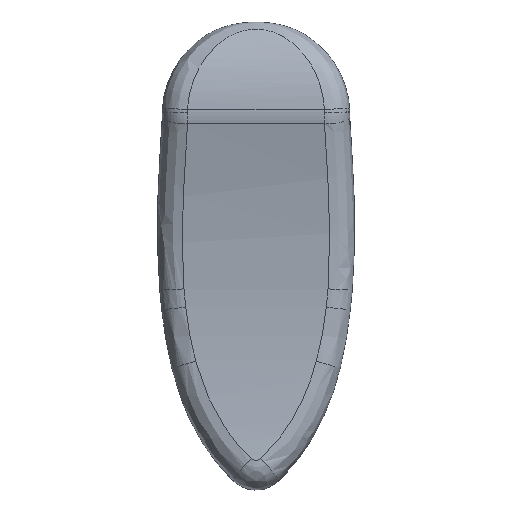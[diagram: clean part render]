
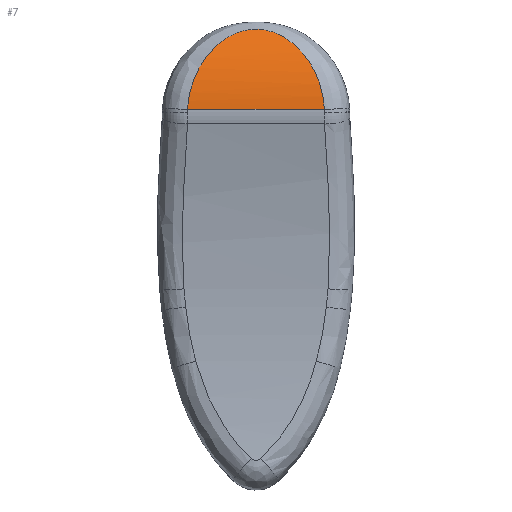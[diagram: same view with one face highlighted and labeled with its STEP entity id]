
A CAD part, top view. The second image highlights one B-rep face of the part: STEP entity #7.
In plain terms, the highlighted free-form (B-spline) face has degree [3, 1] with [4, 2] control points.
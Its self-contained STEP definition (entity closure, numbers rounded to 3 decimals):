
#7 = ADVANCED_FACE ( 'NONE', ( #804 ), #284, .T. ) ;
#9 = CARTESIAN_POINT ( 'NONE',  ( 25.436, 68.469, -62.998 ) ) ;
#22 = CARTESIAN_POINT ( 'NONE',  ( 2.512, 73.556, -64.651 ) ) ;
#30 = CARTESIAN_POINT ( 'NONE',  ( 16.093, 78.932, -67.916 ) ) ;
#35 = CARTESIAN_POINT ( 'NONE',  ( 23.451, 72.791, -64.319 ) ) ;
#46 = CARTESIAN_POINT ( 'NONE',  ( 8.005, 78.404, -67.486 ) ) ;
#100 = CARTESIAN_POINT ( 'NONE',  ( -0.837, 63.623, -62.366 ) ) ;
#114 = CARTESIAN_POINT ( 'NONE',  ( 0.157, 68.907, -63.109 ) ) ;
#131 = CARTESIAN_POINT ( 'NONE',  ( 22.933, 73.569, -64.646 ) ) ;
#135 = CARTESIAN_POINT ( 'NONE',  ( -1., 75.813, -65.048 ) ) ;
#139 = CARTESIAN_POINT ( 'NONE',  ( 21.771, 75.006, -65.341 ) ) ;
#147 = CARTESIAN_POINT ( 'NONE',  ( 26.431, 79.63, -68.522 ) ) ;
#168 = CARTESIAN_POINT ( 'NONE',  ( 5.312, 76.614, -66.253 ) ) ;
#174 = EDGE_CURVE ( 'NONE', #657, #1479, #650, .T. ) ;
#196 = ORIENTED_EDGE ( 'NONE', *, *, #174, .T. ) ;
#230 = ORIENTED_EDGE ( 'NONE', *, *, #1003, .T. ) ;
#237 = CARTESIAN_POINT ( 'NONE',  ( 20.806, 76.003, -65.887 ) ) ;
#256 = CARTESIAN_POINT ( 'NONE',  ( 11.724, 79.459, -68.368 ) ) ;
#281 = CARTESIAN_POINT ( 'NONE',  ( 10.259, 79.204, -68.145 ) ) ;
#284 = B_SPLINE_SURFACE_WITH_KNOTS ( 'NONE', 3, 1, ( 
 ( #831, #147 ),
 ( #135, #1433 ),
 ( #1033, #806 ),
 ( #1062, #907 ) ),
 .UNSPECIFIED., .F., .F., .F.,
 ( 4, 4 ),
 ( 2, 2 ),
 ( 0.236, 0.943 ),
 ( 0., 1. ),
 .UNSPECIFIED. ) ;
#294 = CARTESIAN_POINT ( 'NONE',  ( 10.745, 79.313, -68.24 ) ) ;
#302 = EDGE_LOOP ( 'NONE', ( #230, #196 ) ) ;
#311 = CARTESIAN_POINT ( 'NONE',  ( 4.277, 75.694, -65.701 ) ) ;
#388 = CARTESIAN_POINT ( 'NONE',  ( 25.703, 67.537, -62.809 ) ) ;
#393 = CARTESIAN_POINT ( 'NONE',  ( 8.856, 78.789, -67.796 ) ) ;
#426 = CARTESIAN_POINT ( 'NONE',  ( 19.033, 77.467, -66.804 ) ) ;
#501 = CARTESIAN_POINT ( 'NONE',  ( 0.005, 68.442, -63.004 ) ) ;
#526 = CARTESIAN_POINT ( 'NONE',  ( 26.097, 65.601, -62.517 ) ) ;
#529 = CARTESIAN_POINT ( 'NONE',  ( 26.268, 63.623, -62.366 ) ) ;
#536 = CARTESIAN_POINT ( 'NONE',  ( 5.674, 76.907, -66.439 ) ) ;
#627 = CARTESIAN_POINT ( 'NONE',  ( 22.072, 74.657, -65.164 ) ) ;
#636 = DIRECTION ( 'NONE',  ( 1., 0., 0. ) ) ;
#650 = B_SPLINE_CURVE_WITH_KNOTS ( 'NONE', 3,
 ( #529, #1331, #526, #388, #9, #1397, #1654, #35, #131, #627, #139, #1137, #237, #761, #426, #789, #1406, #1661, #30, #1010, #880, #1058, #1529, #904, #256, #294, #281, #393, #46, #1443, #1589, #536, #168, #311, #1568, #1304, #22, #797, #1552, #665, #1046, #114, #501, #1272, #1431, #1545, #1186, #758 ),
 .UNSPECIFIED., .F., .F.,
 ( 4, 2, 2, 2, 2, 2, 2, 2, 2, 2, 2, 2, 2, 2, 2, 2, 2, 2, 2, 2, 2, 2, 2, 4 ),
 ( 0., 0.003, 0.006, 0.009, 0.012, 0.013, 0.015, 0.018, 0.019, 0.021, 0.022, 0.024, 0.025, 0.027, 0.03, 0.031, 0.033, 0.036, 0.037, 0.039, 0.042, 0.043, 0.045, 0.048 ),
 .UNSPECIFIED. ) ;
#657 = VERTEX_POINT ( 'NONE', #1174 ) ;
#662 = VECTOR ( 'NONE', #636, 1000. ) ;
#665 = CARTESIAN_POINT ( 'NONE',  ( 1.055, 71.132, -63.72 ) ) ;
#758 = CARTESIAN_POINT ( 'NONE',  ( -0.837, 63.623, -62.366 ) ) ;
#761 = CARTESIAN_POINT ( 'NONE',  ( 19.771, 76.924, -66.439 ) ) ;
#789 = CARTESIAN_POINT ( 'NONE',  ( 17.833, 78.168, -67.314 ) ) ;
#797 = CARTESIAN_POINT ( 'NONE',  ( 1.99, 72.773, -64.324 ) ) ;
#804 = FACE_OUTER_BOUND ( 'NONE', #302, .T. ) ;
#806 = CARTESIAN_POINT ( 'NONE',  ( 26.431, 70.085, -62.7 ) ) ;
#831 = CARTESIAN_POINT ( 'NONE',  ( -1., 79.63, -68.522 ) ) ;
#880 = CARTESIAN_POINT ( 'NONE',  ( 14.697, 79.311, -68.238 ) ) ;
#904 = CARTESIAN_POINT ( 'NONE',  ( 12.217, 79.496, -68.401 ) ) ;
#907 = CARTESIAN_POINT ( 'NONE',  ( 26.431, 63.623, -62.366 ) ) ;
#1003 = EDGE_CURVE ( 'NONE', #1479, #657, #1350, .T. ) ;
#1010 = CARTESIAN_POINT ( 'NONE',  ( 15.17, 79.204, -68.145 ) ) ;
#1033 = CARTESIAN_POINT ( 'NONE',  ( -1., 70.085, -62.7 ) ) ;
#1046 = CARTESIAN_POINT ( 'NONE',  ( 0.658, 70.267, -63.453 ) ) ;
#1058 = CARTESIAN_POINT ( 'NONE',  ( 13.72, 79.457, -68.367 ) ) ;
#1062 = CARTESIAN_POINT ( 'NONE',  ( -1., 63.623, -62.366 ) ) ;
#1136 = CARTESIAN_POINT ( 'NONE',  ( -5.831, 63.623, -62.366 ) ) ;
#1137 = CARTESIAN_POINT ( 'NONE',  ( 21.139, 75.679, -65.702 ) ) ;
#1174 = CARTESIAN_POINT ( 'NONE',  ( 26.268, 63.623, -62.366 ) ) ;
#1186 = CARTESIAN_POINT ( 'NONE',  ( -0.79, 64.619, -62.417 ) ) ;
#1272 = CARTESIAN_POINT ( 'NONE',  ( -0.26, 67.504, -62.815 ) ) ;
#1304 = CARTESIAN_POINT ( 'NONE',  ( 2.786, 73.933, -64.82 ) ) ;
#1331 = CARTESIAN_POINT ( 'NONE',  ( 26.221, 64.619, -62.417 ) ) ;
#1350 = LINE ( 'NONE', #1136, #662 ) ;
#1397 = CARTESIAN_POINT ( 'NONE',  ( 24.773, 70.265, -63.453 ) ) ;
#1406 = CARTESIAN_POINT ( 'NONE',  ( 17.417, 78.382, -67.477 ) ) ;
#1431 = CARTESIAN_POINT ( 'NONE',  ( -0.375, 67.03, -62.732 ) ) ;
#1433 = CARTESIAN_POINT ( 'NONE',  ( 26.431, 75.813, -65.048 ) ) ;
#1443 = CARTESIAN_POINT ( 'NONE',  ( 6.807, 77.707, -66.978 ) ) ;
#1479 = VERTEX_POINT ( 'NONE', #100 ) ;
#1529 = CARTESIAN_POINT ( 'NONE',  ( 13.213, 79.496, -68.401 ) ) ;
#1545 = CARTESIAN_POINT ( 'NONE',  ( -0.667, 65.595, -62.516 ) ) ;
#1552 = CARTESIAN_POINT ( 'NONE',  ( 1.744, 72.37, -64.167 ) ) ;
#1568 = CARTESIAN_POINT ( 'NONE',  ( 3.649, 75.023, -65.338 ) ) ;
#1589 = CARTESIAN_POINT ( 'NONE',  ( 6.421, 77.453, -66.801 ) ) ;
#1654 = CARTESIAN_POINT ( 'NONE',  ( 24.377, 71.129, -63.719 ) ) ;
#1661 = CARTESIAN_POINT ( 'NONE',  ( 16.545, 78.765, -67.779 ) ) ;
